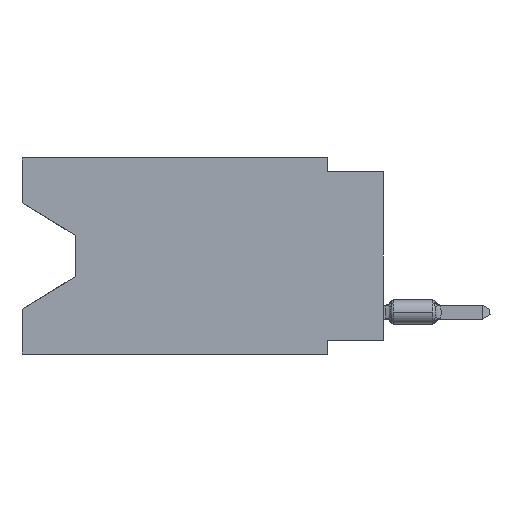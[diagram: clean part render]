
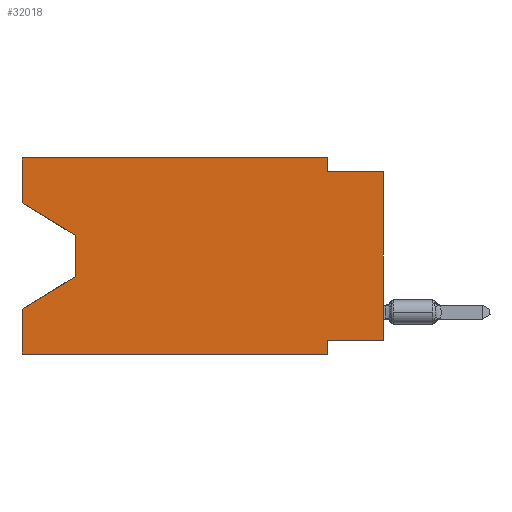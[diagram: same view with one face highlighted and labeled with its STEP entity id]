
A CAD part, left-side view. The second image highlights one B-rep face of the part: STEP entity #32018.
In plain terms, the highlighted planar face has unit normal (-1, 0, 0).
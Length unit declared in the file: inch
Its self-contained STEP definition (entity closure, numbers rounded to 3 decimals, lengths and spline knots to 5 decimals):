
#827 = LINE ( 'NONE', #18267, #28582 ) ;
#937 = DIRECTION ( 'NONE',  ( 0., 0., 1. ) ) ;
#1015 = ORIENTED_EDGE ( 'NONE', *, *, #35841, .T. ) ;
#1104 = VERTEX_POINT ( 'NONE', #19562 ) ;
#1331 = CARTESIAN_POINT ( 'NONE',  ( 0., 0.1, -0.025 ) ) ;
#1516 = LINE ( 'NONE', #21198, #10731 ) ;
#1903 = DIRECTION ( 'NONE',  ( 0., 0., -1. ) ) ;
#2433 = CARTESIAN_POINT ( 'NONE',  ( 0., 0.55, -0.212 ) ) ;
#2792 = CARTESIAN_POINT ( 'NONE',  ( 0., 0., -0.325 ) ) ;
#2935 = VERTEX_POINT ( 'NONE', #25336 ) ;
#2987 = EDGE_CURVE ( 'NONE', #11305, #22035, #14729, .T. ) ;
#3020 = VECTOR ( 'NONE', #6376, 39.37008 ) ;
#3634 = DIRECTION ( 'NONE',  ( 1., 0., 0. ) ) ;
#3827 = ORIENTED_EDGE ( 'NONE', *, *, #8215, .F. ) ;
#5787 = CARTESIAN_POINT ( 'NONE',  ( 0., 0.645, 0. ) ) ;
#5870 = LINE ( 'NONE', #14585, #12663 ) ;
#6376 = DIRECTION ( 'NONE',  ( 0., -1., 0. ) ) ;
#7301 = CARTESIAN_POINT ( 'NONE',  ( 0., 0.1, -0.35 ) ) ;
#7450 = DIRECTION ( 'NONE',  ( 0., -1., 0. ) ) ;
#7537 = ORIENTED_EDGE ( 'NONE', *, *, #9218, .T. ) ;
#8178 = VERTEX_POINT ( 'NONE', #2433 ) ;
#8215 = EDGE_CURVE ( 'NONE', #28352, #10589, #25097, .T. ) ;
#8468 = EDGE_LOOP ( 'NONE', ( #33078, #7537, #8770, #31186, #26845, #16500, #21158, #1015, #31047, #22552, #3827, #9855 ) ) ;
#8770 = ORIENTED_EDGE ( 'NONE', *, *, #19199, .T. ) ;
#9218 = EDGE_CURVE ( 'NONE', #30706, #8178, #21908, .T. ) ;
#9782 = PLANE ( 'NONE',  #26897 ) ;
#9855 = ORIENTED_EDGE ( 'NONE', *, *, #27886, .F. ) ;
#10384 = VERTEX_POINT ( 'NONE', #21500 ) ;
#10589 = VERTEX_POINT ( 'NONE', #25543 ) ;
#10629 = CARTESIAN_POINT ( 'NONE',  ( 0., 0., -0.025 ) ) ;
#10731 = VECTOR ( 'NONE', #7450, 39.37008 ) ;
#11305 = VERTEX_POINT ( 'NONE', #1331 ) ;
#11399 = EDGE_CURVE ( 'NONE', #22117, #1104, #1516, .T. ) ;
#12011 = VECTOR ( 'NONE', #19310, 39.37008 ) ;
#12663 = VECTOR ( 'NONE', #25921, 39.37008 ) ;
#12744 = LINE ( 'NONE', #24060, #27580 ) ;
#12816 = LINE ( 'NONE', #17825, #22986 ) ;
#13036 = EDGE_CURVE ( 'NONE', #10589, #11305, #827, .T. ) ;
#13647 = EDGE_CURVE ( 'NONE', #18349, #27278, #13929, .T. ) ;
#13929 = LINE ( 'NONE', #2792, #18958 ) ;
#13946 = CARTESIAN_POINT ( 'NONE',  ( 0., 0.55, -0.138 ) ) ;
#14167 = CARTESIAN_POINT ( 'NONE',  ( 0., 0., -0.325 ) ) ;
#14585 = CARTESIAN_POINT ( 'NONE',  ( 0., 0.55, -0.212 ) ) ;
#14729 = LINE ( 'NONE', #25881, #3020 ) ;
#15651 = DIRECTION ( 'NONE',  ( 0., 0., -1. ) ) ;
#16198 = LINE ( 'NONE', #7301, #18137 ) ;
#16500 = ORIENTED_EDGE ( 'NONE', *, *, #23121, .F. ) ;
#17448 = VECTOR ( 'NONE', #23253, 39.37008 ) ;
#17675 = LINE ( 'NONE', #20456, #17448 ) ;
#17825 = CARTESIAN_POINT ( 'NONE',  ( 0., 0., 0. ) ) ;
#18137 = VECTOR ( 'NONE', #1903, 39.37008 ) ;
#18267 = CARTESIAN_POINT ( 'NONE',  ( 0., 0.1, 0. ) ) ;
#18349 = VERTEX_POINT ( 'NONE', #14167 ) ;
#18488 = DIRECTION ( 'NONE',  ( 0., -0.855, -0.519 ) ) ;
#18843 = DIRECTION ( 'NONE',  ( 0., 0., -1. ) ) ;
#18958 = VECTOR ( 'NONE', #20049, 39.37008 ) ;
#19199 = EDGE_CURVE ( 'NONE', #8178, #2935, #5870, .T. ) ;
#19310 = DIRECTION ( 'NONE',  ( 0., 0., 1. ) ) ;
#19562 = CARTESIAN_POINT ( 'NONE',  ( 0., 0.1, -0.35 ) ) ;
#20049 = DIRECTION ( 'NONE',  ( 0., 1., 0. ) ) ;
#20168 = EDGE_CURVE ( 'NONE', #22117, #2935, #17675, .T. ) ;
#20456 = CARTESIAN_POINT ( 'NONE',  ( 0., 0.645, 0. ) ) ;
#21082 = CARTESIAN_POINT ( 'NONE',  ( 0., 0.645, 0. ) ) ;
#21158 = ORIENTED_EDGE ( 'NONE', *, *, #13647, .F. ) ;
#21198 = CARTESIAN_POINT ( 'NONE',  ( 0., 0.645, -0.35 ) ) ;
#21500 = CARTESIAN_POINT ( 'NONE',  ( 0., 0.645, -0.08025 ) ) ;
#21901 = CARTESIAN_POINT ( 'NONE',  ( 0., 0.645, 0. ) ) ;
#21908 = LINE ( 'NONE', #13946, #22973 ) ;
#22035 = VERTEX_POINT ( 'NONE', #10629 ) ;
#22117 = VERTEX_POINT ( 'NONE', #25305 ) ;
#22552 = ORIENTED_EDGE ( 'NONE', *, *, #13036, .F. ) ;
#22973 = VECTOR ( 'NONE', #27487, 39.37008 ) ;
#22986 = VECTOR ( 'NONE', #937, 39.37008 ) ;
#23121 = EDGE_CURVE ( 'NONE', #27278, #1104, #16198, .T. ) ;
#23253 = DIRECTION ( 'NONE',  ( 0., 0., 1. ) ) ;
#24060 = CARTESIAN_POINT ( 'NONE',  ( 0., 0.645, -0.08025 ) ) ;
#25097 = LINE ( 'NONE', #5787, #28813 ) ;
#25305 = CARTESIAN_POINT ( 'NONE',  ( 0., 0.645, -0.35 ) ) ;
#25336 = CARTESIAN_POINT ( 'NONE',  ( 0., 0.645, -0.26975 ) ) ;
#25543 = CARTESIAN_POINT ( 'NONE',  ( 0., 0.1, 0. ) ) ;
#25881 = CARTESIAN_POINT ( 'NONE',  ( 0., 0., -0.025 ) ) ;
#25921 = DIRECTION ( 'NONE',  ( 0., 0.855, -0.519 ) ) ;
#26487 = CARTESIAN_POINT ( 'NONE',  ( 0., 0.55, -0.138 ) ) ;
#26845 = ORIENTED_EDGE ( 'NONE', *, *, #11399, .T. ) ;
#26897 = AXIS2_PLACEMENT_3D ( 'NONE', #21082, #3634, #18843 ) ;
#26991 = CARTESIAN_POINT ( 'NONE',  ( 0., 0.1, -0.325 ) ) ;
#27255 = CARTESIAN_POINT ( 'NONE',  ( 0., 0.645, 0. ) ) ;
#27278 = VERTEX_POINT ( 'NONE', #26991 ) ;
#27487 = DIRECTION ( 'NONE',  ( 0., 0., -1. ) ) ;
#27580 = VECTOR ( 'NONE', #18488, 39.37008 ) ;
#27886 = EDGE_CURVE ( 'NONE', #10384, #28352, #30452, .T. ) ;
#28352 = VERTEX_POINT ( 'NONE', #27255 ) ;
#28582 = VECTOR ( 'NONE', #15651, 39.37008 ) ;
#28602 = DIRECTION ( 'NONE',  ( 0., -1., 0. ) ) ;
#28813 = VECTOR ( 'NONE', #28602, 39.37008 ) ;
#30452 = LINE ( 'NONE', #21901, #12011 ) ;
#30706 = VERTEX_POINT ( 'NONE', #26487 ) ;
#31047 = ORIENTED_EDGE ( 'NONE', *, *, #2987, .F. ) ;
#31186 = ORIENTED_EDGE ( 'NONE', *, *, #20168, .F. ) ;
#32018 = ADVANCED_FACE ( 'NONE', ( #35193 ), #9782, .F. ) ;
#33078 = ORIENTED_EDGE ( 'NONE', *, *, #33186, .T. ) ;
#33186 = EDGE_CURVE ( 'NONE', #10384, #30706, #12744, .T. ) ;
#35193 = FACE_OUTER_BOUND ( 'NONE', #8468, .T. ) ;
#35841 = EDGE_CURVE ( 'NONE', #18349, #22035, #12816, .T. ) ;
